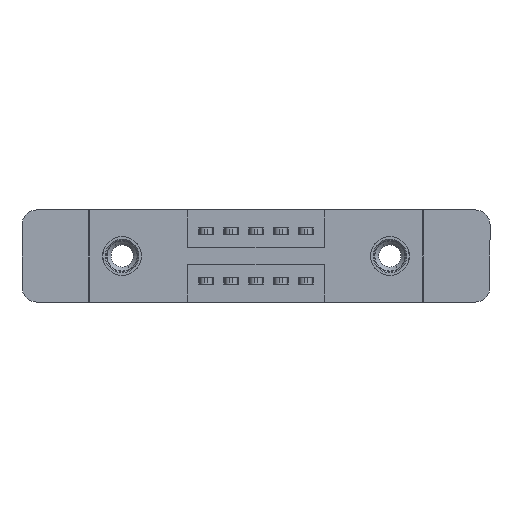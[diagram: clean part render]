
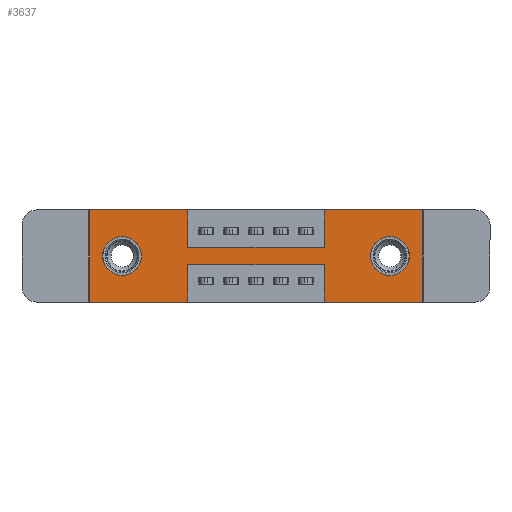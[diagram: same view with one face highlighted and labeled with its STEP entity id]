
A CAD part, front view. The second image highlights one B-rep face of the part: STEP entity #3637.
In plain terms, the highlighted planar face has unit normal (0, -1, 0).
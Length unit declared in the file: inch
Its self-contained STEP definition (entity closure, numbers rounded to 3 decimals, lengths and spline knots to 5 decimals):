
#71 = VERTEX_POINT ( 'NONE', #4355 ) ;
#111 = CARTESIAN_POINT ( 'NONE',  ( 0., 0., -0.37 ) ) ;
#286 = LINE ( 'NONE', #13986, #11959 ) ;
#672 = CARTESIAN_POINT ( 'NONE',  ( 0., 0., 0. ) ) ;
#918 = CARTESIAN_POINT ( 'NONE',  ( 0.13, 0., -0.107 ) ) ;
#1036 = EDGE_CURVE ( 'NONE', #10206, #11241, #10918, .T. ) ;
#1213 = EDGE_CURVE ( 'NONE', #11701, #1996, #6001, .T. ) ;
#1358 = VECTOR ( 'NONE', #8378, 39.37008 ) ;
#1489 = CARTESIAN_POINT ( 'NONE',  ( 1.335, 0., 0. ) ) ;
#1640 = ORIENTED_EDGE ( 'NONE', *, *, #1213, .T. ) ;
#1696 = EDGE_CURVE ( 'NONE', #11241, #3137, #7327, .T. ) ;
#1707 = ORIENTED_EDGE ( 'NONE', *, *, #9487, .F. ) ;
#1747 = ORIENTED_EDGE ( 'NONE', *, *, #8422, .F. ) ;
#1984 = CARTESIAN_POINT ( 'NONE',  ( 0., 0., 0. ) ) ;
#1996 = VERTEX_POINT ( 'NONE', #7048 ) ;
#2053 = FACE_BOUND ( 'NONE', #5690, .T. ) ;
#2174 = CARTESIAN_POINT ( 'NONE',  ( 1.205, 0., -0.107 ) ) ;
#2184 = CARTESIAN_POINT ( 'NONE',  ( 0.9425, 0., -0.37 ) ) ;
#2461 = DIRECTION ( 'NONE',  ( 0., 0., -1. ) ) ;
#2465 = VECTOR ( 'NONE', #5119, 39.37008 ) ;
#2594 = ORIENTED_EDGE ( 'NONE', *, *, #10578, .F. ) ;
#2657 = VECTOR ( 'NONE', #10399, 39.37008 ) ;
#2658 = EDGE_CURVE ( 'NONE', #11309, #10995, #12548, .T. ) ;
#2912 = ORIENTED_EDGE ( 'NONE', *, *, #10628, .T. ) ;
#3137 = VERTEX_POINT ( 'NONE', #5686 ) ;
#3459 = DIRECTION ( 'NONE',  ( 0., -1., 0. ) ) ;
#3479 = VECTOR ( 'NONE', #7185, 39.37008 ) ;
#3585 = CIRCLE ( 'NONE', #3740, 0.078 ) ;
#3637 = ADVANCED_FACE ( 'NONE', ( #2053, #4456, #13216 ), #12025, .T. ) ;
#3740 = AXIS2_PLACEMENT_3D ( 'NONE', #5211, #12659, #10472 ) ;
#3854 = ORIENTED_EDGE ( 'NONE', *, *, #2658, .F. ) ;
#3895 = ORIENTED_EDGE ( 'NONE', *, *, #6797, .F. ) ;
#4064 = VERTEX_POINT ( 'NONE', #4443 ) ;
#4355 = CARTESIAN_POINT ( 'NONE',  ( 0.3925, 0., -0.37 ) ) ;
#4374 = LINE ( 'NONE', #12544, #6204 ) ;
#4414 = VECTOR ( 'NONE', #12686, 39.37008 ) ;
#4443 = CARTESIAN_POINT ( 'NONE',  ( 0.9425, 0., 0. ) ) ;
#4456 = FACE_BOUND ( 'NONE', #10106, .T. ) ;
#4609 = EDGE_CURVE ( 'NONE', #12845, #13852, #3585, .T. ) ;
#4871 = DIRECTION ( 'NONE',  ( 0., 1., 0. ) ) ;
#4914 = DIRECTION ( 'NONE',  ( 0., 1., 0. ) ) ;
#4958 = VECTOR ( 'NONE', #7125, 39.37008 ) ;
#4985 = VERTEX_POINT ( 'NONE', #12454 ) ;
#5108 = EDGE_CURVE ( 'NONE', #10995, #4064, #7748, .T. ) ;
#5119 = DIRECTION ( 'NONE',  ( -1., 0., 0. ) ) ;
#5126 = ORIENTED_EDGE ( 'NONE', *, *, #10916, .T. ) ;
#5211 = CARTESIAN_POINT ( 'NONE',  ( 0.13, 0., -0.185 ) ) ;
#5263 = ORIENTED_EDGE ( 'NONE', *, *, #5108, .F. ) ;
#5442 = LINE ( 'NONE', #10458, #1358 ) ;
#5686 = CARTESIAN_POINT ( 'NONE',  ( 0.9425, 0., -0.22 ) ) ;
#5690 = EDGE_LOOP ( 'NONE', ( #1640, #5126 ) ) ;
#5813 = LINE ( 'NONE', #9478, #9012 ) ;
#5926 = CARTESIAN_POINT ( 'NONE',  ( 1.205, 0., -0.185 ) ) ;
#5938 = CARTESIAN_POINT ( 'NONE',  ( 1.335, 0., -0.37 ) ) ;
#6001 = CIRCLE ( 'NONE', #10563, 0.078 ) ;
#6020 = LINE ( 'NONE', #1984, #2657 ) ;
#6047 = CARTESIAN_POINT ( 'NONE',  ( 0., 0., -0.37 ) ) ;
#6132 = CARTESIAN_POINT ( 'NONE',  ( 1.335, 0., 0. ) ) ;
#6204 = VECTOR ( 'NONE', #12603, 39.37008 ) ;
#6214 = ORIENTED_EDGE ( 'NONE', *, *, #7760, .F. ) ;
#6241 = ORIENTED_EDGE ( 'NONE', *, *, #1696, .F. ) ;
#6265 = CARTESIAN_POINT ( 'NONE',  ( 0.13, 0., -0.185 ) ) ;
#6398 = EDGE_CURVE ( 'NONE', #71, #9153, #286, .T. ) ;
#6558 = CARTESIAN_POINT ( 'NONE',  ( 0.3925, 0., -0.15 ) ) ;
#6763 = CARTESIAN_POINT ( 'NONE',  ( 0., 0., 0. ) ) ;
#6797 = EDGE_CURVE ( 'NONE', #9074, #71, #4374, .T. ) ;
#7048 = CARTESIAN_POINT ( 'NONE',  ( 1.205, 0., -0.263 ) ) ;
#7099 = DIRECTION ( 'NONE',  ( -1., 0., 0. ) ) ;
#7125 = DIRECTION ( 'NONE',  ( 1., 0., 0. ) ) ;
#7133 = CARTESIAN_POINT ( 'NONE',  ( 0.13, 0., -0.263 ) ) ;
#7165 = ORIENTED_EDGE ( 'NONE', *, *, #1036, .F. ) ;
#7185 = DIRECTION ( 'NONE',  ( 1., 0., 0. ) ) ;
#7299 = EDGE_CURVE ( 'NONE', #3137, #9074, #10796, .T. ) ;
#7327 = LINE ( 'NONE', #12154, #10553 ) ;
#7344 = DIRECTION ( 'NONE',  ( 0., 0., 1. ) ) ;
#7356 = ORIENTED_EDGE ( 'NONE', *, *, #7299, .F. ) ;
#7494 = LINE ( 'NONE', #672, #3479 ) ;
#7748 = LINE ( 'NONE', #8232, #4414 ) ;
#7760 = EDGE_CURVE ( 'NONE', #8949, #10206, #12646, .T. ) ;
#8232 = CARTESIAN_POINT ( 'NONE',  ( 0.9425, 0., 0. ) ) ;
#8378 = DIRECTION ( 'NONE',  ( 0., 0., -1. ) ) ;
#8411 = VECTOR ( 'NONE', #7099, 39.37008 ) ;
#8422 = EDGE_CURVE ( 'NONE', #4064, #8949, #6020, .T. ) ;
#8491 = DIRECTION ( 'NONE',  ( -1., 0., 0. ) ) ;
#8701 = ORIENTED_EDGE ( 'NONE', *, *, #6398, .F. ) ;
#8949 = VERTEX_POINT ( 'NONE', #6132 ) ;
#8994 = CIRCLE ( 'NONE', #11374, 0.078 ) ;
#9012 = VECTOR ( 'NONE', #11660, 39.37008 ) ;
#9022 = ORIENTED_EDGE ( 'NONE', *, *, #4609, .T. ) ;
#9074 = VERTEX_POINT ( 'NONE', #11702 ) ;
#9153 = VERTEX_POINT ( 'NONE', #12927 ) ;
#9205 = VERTEX_POINT ( 'NONE', #6763 ) ;
#9314 = CARTESIAN_POINT ( 'NONE',  ( 0.9425, 0., -0.15 ) ) ;
#9478 = CARTESIAN_POINT ( 'NONE',  ( 0., 0., 0. ) ) ;
#9487 = EDGE_CURVE ( 'NONE', #9205, #4985, #7494, .T. ) ;
#9961 = DIRECTION ( 'NONE',  ( 0., 0., 1. ) ) ;
#10106 = EDGE_LOOP ( 'NONE', ( #9022, #2912 ) ) ;
#10206 = VERTEX_POINT ( 'NONE', #5938 ) ;
#10383 = CARTESIAN_POINT ( 'NONE',  ( 0.3925, 0., -0.22 ) ) ;
#10399 = DIRECTION ( 'NONE',  ( 1., 0., 0. ) ) ;
#10458 = CARTESIAN_POINT ( 'NONE',  ( 0.3925, 0., 0. ) ) ;
#10472 = DIRECTION ( 'NONE',  ( 0., 0., 1. ) ) ;
#10496 = CARTESIAN_POINT ( 'NONE',  ( 0.3925, 0., -0.15 ) ) ;
#10553 = VECTOR ( 'NONE', #9961, 39.37008 ) ;
#10563 = AXIS2_PLACEMENT_3D ( 'NONE', #12402, #4914, #12453 ) ;
#10578 = EDGE_CURVE ( 'NONE', #9153, #9205, #5813, .T. ) ;
#10628 = EDGE_CURVE ( 'NONE', #13852, #12845, #11221, .T. ) ;
#10796 = LINE ( 'NONE', #10383, #8411 ) ;
#10916 = EDGE_CURVE ( 'NONE', #1996, #11701, #8994, .T. ) ;
#10918 = LINE ( 'NONE', #6047, #2465 ) ;
#10995 = VERTEX_POINT ( 'NONE', #9314 ) ;
#11221 = CIRCLE ( 'NONE', #13350, 0.078 ) ;
#11241 = VERTEX_POINT ( 'NONE', #2184 ) ;
#11309 = VERTEX_POINT ( 'NONE', #6558 ) ;
#11374 = AXIS2_PLACEMENT_3D ( 'NONE', #5926, #4871, #13580 ) ;
#11660 = DIRECTION ( 'NONE',  ( 0., 0., 1. ) ) ;
#11701 = VERTEX_POINT ( 'NONE', #2174 ) ;
#11702 = CARTESIAN_POINT ( 'NONE',  ( 0.3925, 0., -0.22 ) ) ;
#11959 = VECTOR ( 'NONE', #8491, 39.37008 ) ;
#12025 = PLANE ( 'NONE',  #12490 ) ;
#12154 = CARTESIAN_POINT ( 'NONE',  ( 0.9425, 0., -0.37 ) ) ;
#12309 = DIRECTION ( 'NONE',  ( 0., 0., -1. ) ) ;
#12402 = CARTESIAN_POINT ( 'NONE',  ( 1.205, 0., -0.185 ) ) ;
#12453 = DIRECTION ( 'NONE',  ( 0., 0., -1. ) ) ;
#12454 = CARTESIAN_POINT ( 'NONE',  ( 0.3925, 0., 0. ) ) ;
#12490 = AXIS2_PLACEMENT_3D ( 'NONE', #111, #3459, #2461 ) ;
#12514 = EDGE_LOOP ( 'NONE', ( #3895, #7356, #6241, #7165, #6214, #1747, #5263, #3854, #12636, #1707, #2594, #8701 ) ) ;
#12544 = CARTESIAN_POINT ( 'NONE',  ( 0.3925, 0., -0.37 ) ) ;
#12548 = LINE ( 'NONE', #10496, #4958 ) ;
#12603 = DIRECTION ( 'NONE',  ( 0., 0., -1. ) ) ;
#12636 = ORIENTED_EDGE ( 'NONE', *, *, #12667, .F. ) ;
#12646 = LINE ( 'NONE', #1489, #13998 ) ;
#12659 = DIRECTION ( 'NONE',  ( 0., 1., 0. ) ) ;
#12667 = EDGE_CURVE ( 'NONE', #4985, #11309, #5442, .T. ) ;
#12686 = DIRECTION ( 'NONE',  ( 0., 0., 1. ) ) ;
#12845 = VERTEX_POINT ( 'NONE', #918 ) ;
#12927 = CARTESIAN_POINT ( 'NONE',  ( 0., 0., -0.37 ) ) ;
#13216 = FACE_OUTER_BOUND ( 'NONE', #12514, .T. ) ;
#13350 = AXIS2_PLACEMENT_3D ( 'NONE', #6265, #13836, #7344 ) ;
#13580 = DIRECTION ( 'NONE',  ( 0., 0., -1. ) ) ;
#13836 = DIRECTION ( 'NONE',  ( 0., 1., 0. ) ) ;
#13852 = VERTEX_POINT ( 'NONE', #7133 ) ;
#13986 = CARTESIAN_POINT ( 'NONE',  ( 0., 0., -0.37 ) ) ;
#13998 = VECTOR ( 'NONE', #12309, 39.37008 ) ;
